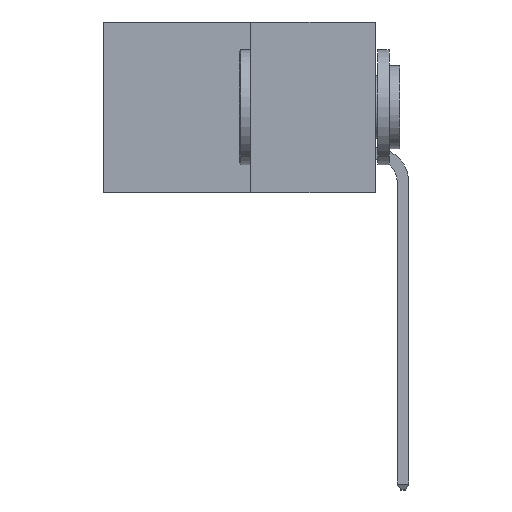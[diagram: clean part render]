
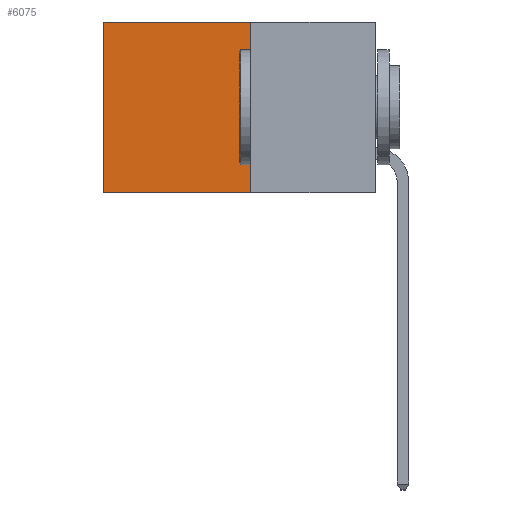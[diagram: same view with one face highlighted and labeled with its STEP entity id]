
A CAD part, left-side view. The second image highlights one B-rep face of the part: STEP entity #6075.
In plain terms, the highlighted planar face has unit normal (-1, 0, 0).
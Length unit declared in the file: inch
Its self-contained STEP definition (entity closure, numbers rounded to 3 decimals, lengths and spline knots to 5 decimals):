
#260 = DIRECTION ( 'NONE',  ( 0., 0., -1. ) ) ;
#297 = DIRECTION ( 'NONE',  ( 1., 0., 0. ) ) ;
#314 = CARTESIAN_POINT ( 'NONE',  ( 0.277, 0.59, -0.37 ) ) ;
#364 = ORIENTED_EDGE ( 'NONE', *, *, #9448, .T. ) ;
#375 = ORIENTED_EDGE ( 'NONE', *, *, #6976, .F. ) ;
#402 = ORIENTED_EDGE ( 'NONE', *, *, #6069, .F. ) ;
#405 = ORIENTED_EDGE ( 'NONE', *, *, #4418, .T. ) ;
#554 = CARTESIAN_POINT ( 'NONE',  ( 0.277, 0.27, -0.37 ) ) ;
#578 = LINE ( 'NONE', #8407, #7204 ) ;
#1091 = LINE ( 'NONE', #10609, #5455 ) ;
#1139 = DIRECTION ( 'NONE',  ( 0., 0., -1. ) ) ;
#1175 = CARTESIAN_POINT ( 'NONE',  ( 0.277, 0.27, -0.37 ) ) ;
#1184 = PLANE ( 'NONE',  #2064 ) ;
#1441 = VERTEX_POINT ( 'NONE', #314 ) ;
#1448 = VECTOR ( 'NONE', #1139, 39.37008 ) ;
#2064 = AXIS2_PLACEMENT_3D ( 'NONE', #1175, #297, #260 ) ;
#3173 = EDGE_LOOP ( 'NONE', ( #364, #375, #402, #405 ) ) ;
#3267 = VERTEX_POINT ( 'NONE', #3706 ) ;
#3706 = CARTESIAN_POINT ( 'NONE',  ( 0.277, 0.27, 0. ) ) ;
#4009 = LINE ( 'NONE', #554, #1448 ) ;
#4418 = EDGE_CURVE ( 'NONE', #3267, #5117, #1091, .T. ) ;
#5117 = VERTEX_POINT ( 'NONE', #9452 ) ;
#5455 = VECTOR ( 'NONE', #10690, 39.37008 ) ;
#6041 = FACE_OUTER_BOUND ( 'NONE', #3173, .T. ) ;
#6069 = EDGE_CURVE ( 'NONE', #3267, #6989, #4009, .T. ) ;
#6075 = ADVANCED_FACE ( 'NONE', ( #6041 ), #1184, .F. ) ;
#6543 = CARTESIAN_POINT ( 'NONE',  ( 0.277, 0.59, -0.37 ) ) ;
#6871 = LINE ( 'NONE', #6543, #8580 ) ;
#6976 = EDGE_CURVE ( 'NONE', #6989, #1441, #578, .T. ) ;
#6989 = VERTEX_POINT ( 'NONE', #8311 ) ;
#7204 = VECTOR ( 'NONE', #8435, 39.37008 ) ;
#8311 = CARTESIAN_POINT ( 'NONE',  ( 0.277, 0.27, -0.37 ) ) ;
#8407 = CARTESIAN_POINT ( 'NONE',  ( 0.277, 0.27, -0.37 ) ) ;
#8435 = DIRECTION ( 'NONE',  ( 0., 1., 0. ) ) ;
#8580 = VECTOR ( 'NONE', #10514, 39.37008 ) ;
#9448 = EDGE_CURVE ( 'NONE', #5117, #1441, #6871, .T. ) ;
#9452 = CARTESIAN_POINT ( 'NONE',  ( 0.277, 0.59, 0. ) ) ;
#10514 = DIRECTION ( 'NONE',  ( 0., 0., -1. ) ) ;
#10609 = CARTESIAN_POINT ( 'NONE',  ( 0.277, 0.27, 0. ) ) ;
#10690 = DIRECTION ( 'NONE',  ( 0., 1., 0. ) ) ;
